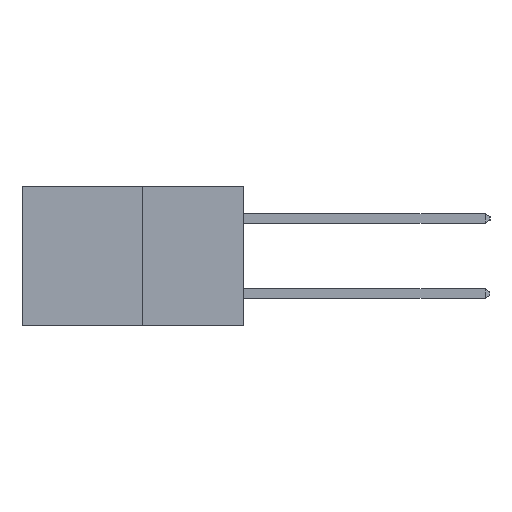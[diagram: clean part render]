
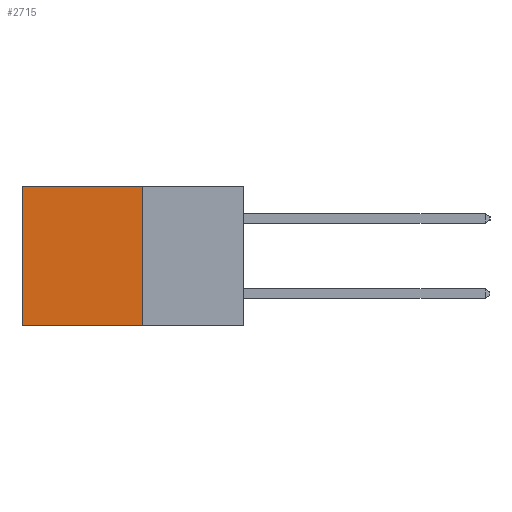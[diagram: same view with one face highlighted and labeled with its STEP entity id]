
A CAD part, left-side view. The second image highlights one B-rep face of the part: STEP entity #2715.
In plain terms, the highlighted planar face has unit normal (-1, 0, 0).
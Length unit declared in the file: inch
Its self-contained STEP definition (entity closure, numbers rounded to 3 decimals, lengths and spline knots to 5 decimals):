
#165 = DIRECTION ( 'NONE',  ( 0., 0., -1. ) ) ;
#169 = CARTESIAN_POINT ( 'NONE',  ( 0.277, 0.27, -0.37 ) ) ;
#719 = CARTESIAN_POINT ( 'NONE',  ( 0.277, 0.59, -0.37 ) ) ;
#799 = CARTESIAN_POINT ( 'NONE',  ( 0.277, 0.27, -0.37 ) ) ;
#1186 = VERTEX_POINT ( 'NONE', #4362 ) ;
#1240 = CARTESIAN_POINT ( 'NONE',  ( 0.277, 0.59, 0. ) ) ;
#1316 = DIRECTION ( 'NONE',  ( 0., 1., 0. ) ) ;
#1435 = VECTOR ( 'NONE', #9457, 39.37008 ) ;
#1747 = CARTESIAN_POINT ( 'NONE',  ( 0.277, 0.27, 0. ) ) ;
#1974 = VECTOR ( 'NONE', #2498, 39.37008 ) ;
#2065 = VERTEX_POINT ( 'NONE', #1240 ) ;
#2327 = VECTOR ( 'NONE', #1316, 39.37008 ) ;
#2498 = DIRECTION ( 'NONE',  ( 0., 1., 0. ) ) ;
#2556 = CARTESIAN_POINT ( 'NONE',  ( 0.277, 0.27, -0.37 ) ) ;
#2715 = ADVANCED_FACE ( 'NONE', ( #8540 ), #3954, .F. ) ;
#2958 = AXIS2_PLACEMENT_3D ( 'NONE', #3935, #3899, #3887 ) ;
#3406 = CARTESIAN_POINT ( 'NONE',  ( 0.277, 0.59, -0.37 ) ) ;
#3730 = EDGE_CURVE ( 'NONE', #6705, #4836, #7959, .T. ) ;
#3887 = DIRECTION ( 'NONE',  ( 0., 0., -1. ) ) ;
#3899 = DIRECTION ( 'NONE',  ( 1., 0., 0. ) ) ;
#3935 = CARTESIAN_POINT ( 'NONE',  ( 0.277, 0.27, -0.37 ) ) ;
#3954 = PLANE ( 'NONE',  #2958 ) ;
#4362 = CARTESIAN_POINT ( 'NONE',  ( 0.277, 0.27, 0. ) ) ;
#4513 = VECTOR ( 'NONE', #165, 39.37008 ) ;
#4573 = EDGE_CURVE ( 'NONE', #1186, #6705, #6244, .T. ) ;
#4836 = VERTEX_POINT ( 'NONE', #3406 ) ;
#5041 = EDGE_LOOP ( 'NONE', ( #5683, #5535, #5337, #8807 ) ) ;
#5337 = ORIENTED_EDGE ( 'NONE', *, *, #4573, .F. ) ;
#5535 = ORIENTED_EDGE ( 'NONE', *, *, #3730, .F. ) ;
#5683 = ORIENTED_EDGE ( 'NONE', *, *, #5766, .T. ) ;
#5766 = EDGE_CURVE ( 'NONE', #2065, #4836, #7334, .T. ) ;
#6244 = LINE ( 'NONE', #169, #4513 ) ;
#6705 = VERTEX_POINT ( 'NONE', #2556 ) ;
#7334 = LINE ( 'NONE', #719, #1435 ) ;
#7841 = LINE ( 'NONE', #1747, #1974 ) ;
#7959 = LINE ( 'NONE', #799, #2327 ) ;
#8082 = EDGE_CURVE ( 'NONE', #1186, #2065, #7841, .T. ) ;
#8540 = FACE_OUTER_BOUND ( 'NONE', #5041, .T. ) ;
#8807 = ORIENTED_EDGE ( 'NONE', *, *, #8082, .T. ) ;
#9457 = DIRECTION ( 'NONE',  ( 0., 0., -1. ) ) ;
